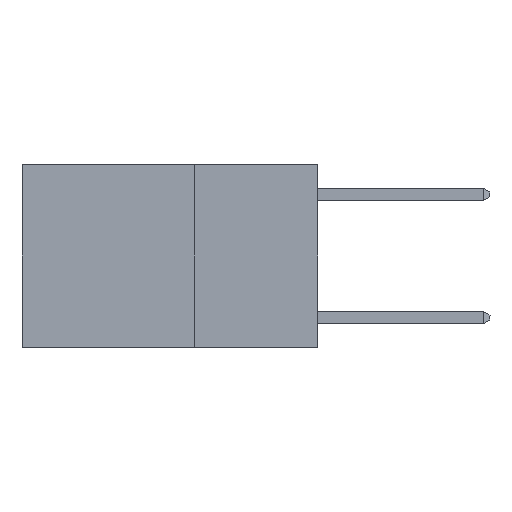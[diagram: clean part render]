
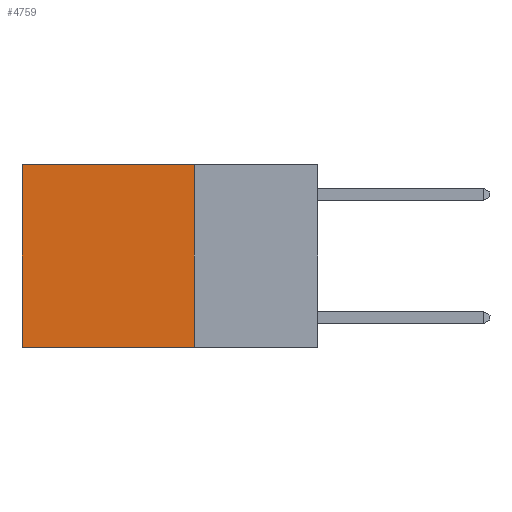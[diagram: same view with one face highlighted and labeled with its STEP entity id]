
A CAD part, left-side view. The second image highlights one B-rep face of the part: STEP entity #4759.
In plain terms, the highlighted planar face has unit normal (-1, 0, 0).
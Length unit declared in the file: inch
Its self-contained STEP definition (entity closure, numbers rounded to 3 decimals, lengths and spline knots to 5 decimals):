
#54 = CARTESIAN_POINT ( 'NONE',  ( 0.2625, 0.25, -0.37 ) ) ;
#159 = DIRECTION ( 'NONE',  ( 1., 0., 0. ) ) ;
#742 = FACE_OUTER_BOUND ( 'NONE', #797, .T. ) ;
#789 = DIRECTION ( 'NONE',  ( 0., 0., -1. ) ) ;
#797 = EDGE_LOOP ( 'NONE', ( #6809, #8459, #6936, #8789 ) ) ;
#1023 = VECTOR ( 'NONE', #4871, 39.37008 ) ;
#1170 = VERTEX_POINT ( 'NONE', #1887 ) ;
#1269 = LINE ( 'NONE', #54, #1023 ) ;
#1308 = DIRECTION ( 'NONE',  ( 0., 0., -1. ) ) ;
#1434 = EDGE_CURVE ( 'NONE', #1170, #9344, #8625, .T. ) ;
#1449 = CARTESIAN_POINT ( 'NONE',  ( 0.2625, 0.25, 0. ) ) ;
#1614 = CARTESIAN_POINT ( 'NONE',  ( 0.2625, 0.6, 0. ) ) ;
#1675 = CARTESIAN_POINT ( 'NONE',  ( 0.2625, 0.25, 0. ) ) ;
#1726 = CARTESIAN_POINT ( 'NONE',  ( 0.2625, 0.6, -0.37 ) ) ;
#1887 = CARTESIAN_POINT ( 'NONE',  ( 0.2625, 0.25, 0. ) ) ;
#2324 = EDGE_CURVE ( 'NONE', #9344, #7826, #1269, .T. ) ;
#2697 = VECTOR ( 'NONE', #1308, 39.37008 ) ;
#2803 = VECTOR ( 'NONE', #7019, 39.37008 ) ;
#3235 = PLANE ( 'NONE',  #7579 ) ;
#3857 = CARTESIAN_POINT ( 'NONE',  ( 0.2625, 0.6, 0. ) ) ;
#4264 = LINE ( 'NONE', #3857, #9589 ) ;
#4387 = CARTESIAN_POINT ( 'NONE',  ( 0.2625, 0.25, -0.37 ) ) ;
#4687 = VERTEX_POINT ( 'NONE', #1614 ) ;
#4748 = EDGE_CURVE ( 'NONE', #1170, #4687, #8924, .T. ) ;
#4759 = ADVANCED_FACE ( 'NONE', ( #742 ), #3235, .F. ) ;
#4871 = DIRECTION ( 'NONE',  ( 0., 1., 0. ) ) ;
#5556 = DIRECTION ( 'NONE',  ( 0., 0., -1. ) ) ;
#6296 = CARTESIAN_POINT ( 'NONE',  ( 0.2625, 0.25, 0. ) ) ;
#6809 = ORIENTED_EDGE ( 'NONE', *, *, #9534, .T. ) ;
#6936 = ORIENTED_EDGE ( 'NONE', *, *, #1434, .F. ) ;
#7019 = DIRECTION ( 'NONE',  ( 0., 1., 0. ) ) ;
#7579 = AXIS2_PLACEMENT_3D ( 'NONE', #1675, #159, #5556 ) ;
#7826 = VERTEX_POINT ( 'NONE', #1726 ) ;
#8459 = ORIENTED_EDGE ( 'NONE', *, *, #2324, .F. ) ;
#8625 = LINE ( 'NONE', #1449, #2697 ) ;
#8789 = ORIENTED_EDGE ( 'NONE', *, *, #4748, .T. ) ;
#8924 = LINE ( 'NONE', #6296, #2803 ) ;
#9344 = VERTEX_POINT ( 'NONE', #4387 ) ;
#9534 = EDGE_CURVE ( 'NONE', #4687, #7826, #4264, .T. ) ;
#9589 = VECTOR ( 'NONE', #789, 39.37008 ) ;
